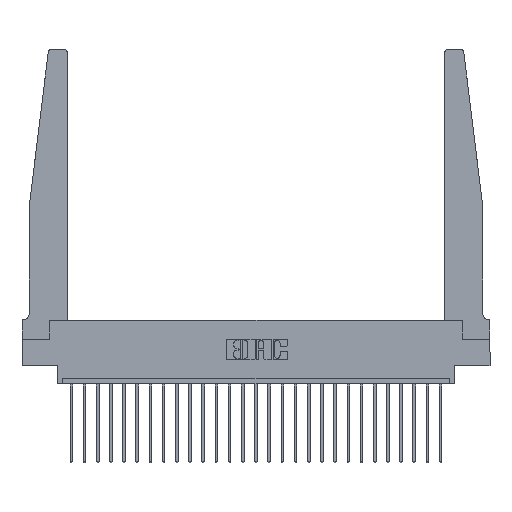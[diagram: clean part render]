
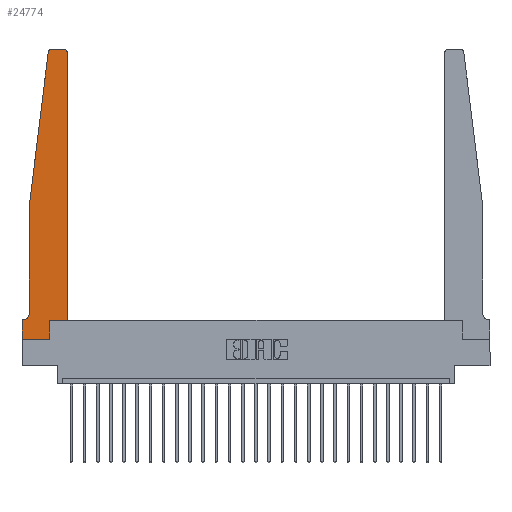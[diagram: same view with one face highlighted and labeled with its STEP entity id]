
A CAD part, top view. The second image highlights one B-rep face of the part: STEP entity #24774.
In plain terms, the highlighted planar face has unit normal (0, 0, 1).
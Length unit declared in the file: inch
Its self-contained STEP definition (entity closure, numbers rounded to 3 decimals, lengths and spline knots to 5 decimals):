
#289 = ORIENTED_EDGE ( 'NONE', *, *, #19366, .T. ) ;
#314 = EDGE_CURVE ( 'NONE', #19261, #17080, #16512, .T. ) ;
#381 = DIRECTION ( 'NONE',  ( 0., 0., 1. ) ) ;
#766 = CARTESIAN_POINT ( 'NONE',  ( 0.27653, 2.72, 0.37 ) ) ;
#783 = FACE_OUTER_BOUND ( 'NONE', #7687, .T. ) ;
#830 = CARTESIAN_POINT ( 'NONE',  ( 0.425, 0.18, 0.37 ) ) ;
#916 = LINE ( 'NONE', #3320, #4278 ) ;
#1027 = VERTEX_POINT ( 'NONE', #17468 ) ;
#1096 = DIRECTION ( 'NONE',  ( 0., -1., 0. ) ) ;
#1264 = CARTESIAN_POINT ( 'NONE',  ( 0.425, 0.18, 0.37 ) ) ;
#1485 = ORIENTED_EDGE ( 'NONE', *, *, #8871, .T. ) ;
#1507 = AXIS2_PLACEMENT_3D ( 'NONE', #21925, #4410, #5948 ) ;
#2070 = CARTESIAN_POINT ( 'NONE',  ( 0.24675, 2.72367, 0.37 ) ) ;
#2251 = VECTOR ( 'NONE', #10644, 39.37008 ) ;
#2255 = VECTOR ( 'NONE', #1096, 39.37008 ) ;
#2747 = LINE ( 'NONE', #22167, #2255 ) ;
#3196 = DIRECTION ( 'NONE',  ( 1., 0., 0. ) ) ;
#3212 = VERTEX_POINT ( 'NONE', #16031 ) ;
#3320 = CARTESIAN_POINT ( 'NONE',  ( 0.065, 1.25, 0.37 ) ) ;
#3847 = LINE ( 'NONE', #23647, #10254 ) ;
#4278 = VECTOR ( 'NONE', #20333, 39.37008 ) ;
#4377 = EDGE_CURVE ( 'NONE', #4776, #20183, #16183, .T. ) ;
#4410 = DIRECTION ( 'NONE',  ( 0., 0., -1. ) ) ;
#4450 = EDGE_CURVE ( 'NONE', #18520, #14397, #2747, .T. ) ;
#4516 = ORIENTED_EDGE ( 'NONE', *, *, #11067, .T. ) ;
#4520 = DIRECTION ( 'NONE',  ( 1., 0., 0. ) ) ;
#4776 = VERTEX_POINT ( 'NONE', #9916 ) ;
#5104 = CARTESIAN_POINT ( 'NONE',  ( 0.065, 1.25, 0.37 ) ) ;
#5948 = DIRECTION ( 'NONE',  ( -1., 0., 0. ) ) ;
#6250 = DIRECTION ( 'NONE',  ( 0., -1., 0. ) ) ;
#6401 = ORIENTED_EDGE ( 'NONE', *, *, #9614, .T. ) ;
#6739 = PLANE ( 'NONE',  #21978 ) ;
#7006 = EDGE_CURVE ( 'NONE', #3212, #23876, #16461, .T. ) ;
#7345 = EDGE_CURVE ( 'NONE', #11373, #4776, #19206, .T. ) ;
#7687 = EDGE_LOOP ( 'NONE', ( #4516, #14678, #1485, #21021, #6401, #15862, #289, #20171, #20343, #18769, #23490, #15819 ) ) ;
#7941 = AXIS2_PLACEMENT_3D ( 'NONE', #21776, #8063, #11843 ) ;
#8063 = DIRECTION ( 'NONE',  ( 0., 0., 1. ) ) ;
#8176 = VECTOR ( 'NONE', #4520, 39.37008 ) ;
#8824 = CARTESIAN_POINT ( 'NONE',  ( 0., 0.1875, 0.37 ) ) ;
#8871 = EDGE_CURVE ( 'NONE', #11452, #18520, #916, .T. ) ;
#9062 = VECTOR ( 'NONE', #17078, 39.37008 ) ;
#9614 = EDGE_CURVE ( 'NONE', #14397, #19261, #21370, .T. ) ;
#9680 = DIRECTION ( 'NONE',  ( 0., 1., 0. ) ) ;
#9916 = CARTESIAN_POINT ( 'NONE',  ( 0.2605, 0.18, 0.37 ) ) ;
#10105 = CARTESIAN_POINT ( 'NONE',  ( 0., 0., 0.37 ) ) ;
#10254 = VECTOR ( 'NONE', #6250, 39.37008 ) ;
#10644 = DIRECTION ( 'NONE',  ( 0., 1., 0. ) ) ;
#11067 = EDGE_CURVE ( 'NONE', #23876, #15361, #21277, .T. ) ;
#11373 = VERTEX_POINT ( 'NONE', #18456 ) ;
#11452 = VERTEX_POINT ( 'NONE', #2070 ) ;
#11843 = DIRECTION ( 'NONE',  ( 1., 0., 0. ) ) ;
#11946 = EDGE_CURVE ( 'NONE', #1027, #11373, #14289, .T. ) ;
#12545 = CARTESIAN_POINT ( 'NONE',  ( 0.065, 0.2375, 0.37 ) ) ;
#12564 = DIRECTION ( 'NONE',  ( 0., 0., 1. ) ) ;
#12743 = DIRECTION ( 'NONE',  ( 1., 0., 0. ) ) ;
#13800 = CARTESIAN_POINT ( 'NONE',  ( 0.27653, 2.75, 0.37 ) ) ;
#14212 = CARTESIAN_POINT ( 'NONE',  ( 0.425, 0.18, 0.37 ) ) ;
#14222 = EDGE_CURVE ( 'NONE', #15361, #11452, #20773, .T. ) ;
#14289 = LINE ( 'NONE', #10105, #8176 ) ;
#14397 = VERTEX_POINT ( 'NONE', #12545 ) ;
#14591 = DIRECTION ( 'NONE',  ( -1., 0., 0. ) ) ;
#14678 = ORIENTED_EDGE ( 'NONE', *, *, #14222, .T. ) ;
#15141 = CARTESIAN_POINT ( 'NONE',  ( 0.2605, 0.18, 0.37 ) ) ;
#15361 = VERTEX_POINT ( 'NONE', #13800 ) ;
#15682 = CARTESIAN_POINT ( 'NONE',  ( 0.25, 2.75, 0.37 ) ) ;
#15819 = ORIENTED_EDGE ( 'NONE', *, *, #7006, .T. ) ;
#15862 = ORIENTED_EDGE ( 'NONE', *, *, #314, .T. ) ;
#15865 = VECTOR ( 'NONE', #14591, 39.37008 ) ;
#16031 = CARTESIAN_POINT ( 'NONE',  ( 0.425, 2.72, 0.37 ) ) ;
#16041 = VECTOR ( 'NONE', #9680, 39.37008 ) ;
#16183 = LINE ( 'NONE', #830, #22933 ) ;
#16461 = CIRCLE ( 'NONE', #7941, 0.03 ) ;
#16512 = LINE ( 'NONE', #24268, #15865 ) ;
#16518 = CARTESIAN_POINT ( 'NONE',  ( 0., 0.1875, 0.37 ) ) ;
#17078 = DIRECTION ( 'NONE',  ( -1., 0., 0. ) ) ;
#17080 = VERTEX_POINT ( 'NONE', #8824 ) ;
#17468 = CARTESIAN_POINT ( 'NONE',  ( 0., 0., 0.37 ) ) ;
#18456 = CARTESIAN_POINT ( 'NONE',  ( 0.2605, 0., 0.37 ) ) ;
#18520 = VERTEX_POINT ( 'NONE', #5104 ) ;
#18769 = ORIENTED_EDGE ( 'NONE', *, *, #4377, .T. ) ;
#18846 = CARTESIAN_POINT ( 'NONE',  ( 0.015, 0.1875, 0.37 ) ) ;
#19137 = AXIS2_PLACEMENT_3D ( 'NONE', #766, #381, #21584 ) ;
#19206 = LINE ( 'NONE', #15141, #16041 ) ;
#19261 = VERTEX_POINT ( 'NONE', #18846 ) ;
#19366 = EDGE_CURVE ( 'NONE', #17080, #1027, #3847, .T. ) ;
#20171 = ORIENTED_EDGE ( 'NONE', *, *, #11946, .T. ) ;
#20183 = VERTEX_POINT ( 'NONE', #1264 ) ;
#20333 = DIRECTION ( 'NONE',  ( -0.122, -0.992, 0. ) ) ;
#20343 = ORIENTED_EDGE ( 'NONE', *, *, #7345, .T. ) ;
#20773 = CIRCLE ( 'NONE', #19137, 0.03 ) ;
#21021 = ORIENTED_EDGE ( 'NONE', *, *, #4450, .T. ) ;
#21277 = LINE ( 'NONE', #15682, #9062 ) ;
#21370 = CIRCLE ( 'NONE', #1507, 0.05 ) ;
#21584 = DIRECTION ( 'NONE',  ( 1., 0., 0. ) ) ;
#21776 = CARTESIAN_POINT ( 'NONE',  ( 0.395, 2.72, 0.37 ) ) ;
#21819 = CARTESIAN_POINT ( 'NONE',  ( 0.395, 2.75, 0.37 ) ) ;
#21925 = CARTESIAN_POINT ( 'NONE',  ( 0.015, 0.2375, 0.37 ) ) ;
#21978 = AXIS2_PLACEMENT_3D ( 'NONE', #16518, #12564, #3196 ) ;
#22167 = CARTESIAN_POINT ( 'NONE',  ( 0.065, 1.25, 0.37 ) ) ;
#22343 = LINE ( 'NONE', #14212, #2251 ) ;
#22933 = VECTOR ( 'NONE', #12743, 39.37008 ) ;
#23490 = ORIENTED_EDGE ( 'NONE', *, *, #23518, .T. ) ;
#23518 = EDGE_CURVE ( 'NONE', #20183, #3212, #22343, .T. ) ;
#23647 = CARTESIAN_POINT ( 'NONE',  ( 0., 0., 0.37 ) ) ;
#23876 = VERTEX_POINT ( 'NONE', #21819 ) ;
#24268 = CARTESIAN_POINT ( 'NONE',  ( 0.065, 0.1875, 0.37 ) ) ;
#24774 = ADVANCED_FACE ( 'NONE', ( #783 ), #6739, .T. ) ;
